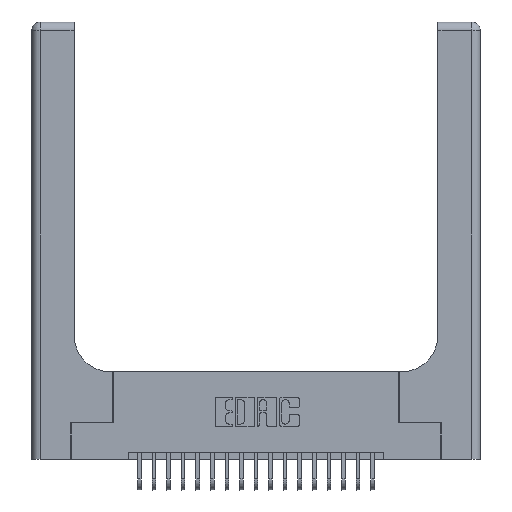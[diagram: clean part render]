
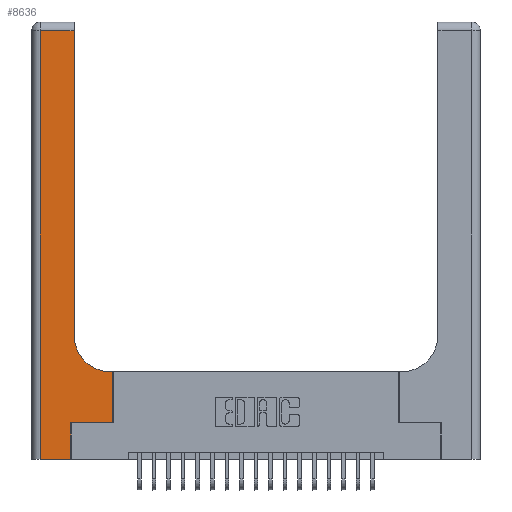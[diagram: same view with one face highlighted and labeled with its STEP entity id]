
A CAD part, top view. The second image highlights one B-rep face of the part: STEP entity #8636.
In plain terms, the highlighted planar face has unit normal (0, 0, 1).
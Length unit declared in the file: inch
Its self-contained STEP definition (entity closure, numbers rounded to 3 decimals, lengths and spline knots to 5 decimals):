
#656 = EDGE_CURVE ( 'NONE', #9086, #6946, #1847, .T. ) ;
#853 = VERTEX_POINT ( 'NONE', #21375 ) ;
#895 = CARTESIAN_POINT ( 'NONE',  ( 0.269, 0., 0.37 ) ) ;
#916 = LINE ( 'NONE', #15153, #19738 ) ;
#1081 = LINE ( 'NONE', #7070, #23276 ) ;
#1116 = VERTEX_POINT ( 'NONE', #2215 ) ;
#1467 = VECTOR ( 'NONE', #8003, 39.37008 ) ;
#1506 = VECTOR ( 'NONE', #14031, 39.37008 ) ;
#1847 = LINE ( 'NONE', #6470, #15522 ) ;
#2215 = CARTESIAN_POINT ( 'NONE',  ( 0.2915, 2.94, 0.37 ) ) ;
#2321 = DIRECTION ( 'NONE',  ( 0., 0., -1. ) ) ;
#2391 = DIRECTION ( 'NONE',  ( 0., 0., -1. ) ) ;
#2505 = EDGE_CURVE ( 'NONE', #12553, #1116, #916, .T. ) ;
#2933 = LINE ( 'NONE', #3428, #1506 ) ;
#3012 = ORIENTED_EDGE ( 'NONE', *, *, #11984, .T. ) ;
#3163 = EDGE_CURVE ( 'NONE', #1116, #22739, #12796, .T. ) ;
#3407 = CARTESIAN_POINT ( 'NONE',  ( 0.2915, 0.85, 0.37 ) ) ;
#3428 = CARTESIAN_POINT ( 'NONE',  ( 0., 0., 0.37 ) ) ;
#4200 = CARTESIAN_POINT ( 'NONE',  ( 0.5585, 0.25, 0.37 ) ) ;
#4352 = EDGE_CURVE ( 'NONE', #22739, #20454, #1081, .T. ) ;
#4397 = LINE ( 'NONE', #4946, #15492 ) ;
#4946 = CARTESIAN_POINT ( 'NONE',  ( 0.2915, 0.6, 0.37 ) ) ;
#6448 = ORIENTED_EDGE ( 'NONE', *, *, #22665, .T. ) ;
#6470 = CARTESIAN_POINT ( 'NONE',  ( 0.269, 0.25, 0.37 ) ) ;
#6734 = CARTESIAN_POINT ( 'NONE',  ( 0., 2.94, 0.37 ) ) ;
#6946 = VERTEX_POINT ( 'NONE', #21817 ) ;
#7070 = CARTESIAN_POINT ( 'NONE',  ( 0.06, 3., 0.37 ) ) ;
#7709 = LINE ( 'NONE', #4200, #1467 ) ;
#7844 = CARTESIAN_POINT ( 'NONE',  ( 0.269, 0., 0.37 ) ) ;
#7920 = EDGE_CURVE ( 'NONE', #6946, #853, #7709, .T. ) ;
#8003 = DIRECTION ( 'NONE',  ( 0., 1., 0. ) ) ;
#8152 = AXIS2_PLACEMENT_3D ( 'NONE', #13316, #2391, #16904 ) ;
#8636 = ADVANCED_FACE ( 'NONE', ( #13153 ), #13398, .F. ) ;
#8819 = DIRECTION ( 'NONE',  ( 0., -1., 0. ) ) ;
#9086 = VERTEX_POINT ( 'NONE', #16178 ) ;
#9945 = VERTEX_POINT ( 'NONE', #16929 ) ;
#10092 = CIRCLE ( 'NONE', #14457, 0.25 ) ;
#10537 = ORIENTED_EDGE ( 'NONE', *, *, #7920, .T. ) ;
#10909 = CARTESIAN_POINT ( 'NONE',  ( 0.06, 2.94, 0.37 ) ) ;
#11194 = DIRECTION ( 'NONE',  ( 1., 0., 0. ) ) ;
#11984 = EDGE_CURVE ( 'NONE', #20454, #20222, #2933, .T. ) ;
#12553 = VERTEX_POINT ( 'NONE', #3407 ) ;
#12619 = ORIENTED_EDGE ( 'NONE', *, *, #4352, .T. ) ;
#12796 = LINE ( 'NONE', #6734, #16226 ) ;
#13107 = EDGE_LOOP ( 'NONE', ( #14057, #20870, #12619, #3012, #14576, #21578, #10537, #6448, #15050 ) ) ;
#13153 = FACE_OUTER_BOUND ( 'NONE', #13107, .T. ) ;
#13316 = CARTESIAN_POINT ( 'NONE',  ( 0., 3., 0.37 ) ) ;
#13398 = PLANE ( 'NONE',  #8152 ) ;
#14031 = DIRECTION ( 'NONE',  ( 1., 0., 0. ) ) ;
#14057 = ORIENTED_EDGE ( 'NONE', *, *, #2505, .T. ) ;
#14151 = EDGE_CURVE ( 'NONE', #20222, #9086, #19675, .T. ) ;
#14457 = AXIS2_PLACEMENT_3D ( 'NONE', #18667, #2321, #11194 ) ;
#14576 = ORIENTED_EDGE ( 'NONE', *, *, #14151, .T. ) ;
#15050 = ORIENTED_EDGE ( 'NONE', *, *, #22252, .T. ) ;
#15153 = CARTESIAN_POINT ( 'NONE',  ( 0.2915, 3., 0.37 ) ) ;
#15492 = VECTOR ( 'NONE', #17702, 39.37008 ) ;
#15522 = VECTOR ( 'NONE', #22876, 39.37008 ) ;
#16178 = CARTESIAN_POINT ( 'NONE',  ( 0.269, 0.25, 0.37 ) ) ;
#16226 = VECTOR ( 'NONE', #17577, 39.37008 ) ;
#16904 = DIRECTION ( 'NONE',  ( -1., 0., 0. ) ) ;
#16929 = CARTESIAN_POINT ( 'NONE',  ( 0.5415, 0.6, 0.37 ) ) ;
#17378 = VECTOR ( 'NONE', #19132, 39.37008 ) ;
#17577 = DIRECTION ( 'NONE',  ( -1., 0., 0. ) ) ;
#17702 = DIRECTION ( 'NONE',  ( -1., 0., 0. ) ) ;
#18111 = CARTESIAN_POINT ( 'NONE',  ( 0.06, 0., 0.37 ) ) ;
#18667 = CARTESIAN_POINT ( 'NONE',  ( 0.5415, 0.85, 0.37 ) ) ;
#18822 = DIRECTION ( 'NONE',  ( 0., 1., 0. ) ) ;
#19132 = DIRECTION ( 'NONE',  ( 0., 1., 0. ) ) ;
#19675 = LINE ( 'NONE', #895, #17378 ) ;
#19738 = VECTOR ( 'NONE', #18822, 39.37008 ) ;
#20222 = VERTEX_POINT ( 'NONE', #7844 ) ;
#20454 = VERTEX_POINT ( 'NONE', #18111 ) ;
#20870 = ORIENTED_EDGE ( 'NONE', *, *, #3163, .T. ) ;
#21375 = CARTESIAN_POINT ( 'NONE',  ( 0.5585, 0.6, 0.37 ) ) ;
#21578 = ORIENTED_EDGE ( 'NONE', *, *, #656, .T. ) ;
#21817 = CARTESIAN_POINT ( 'NONE',  ( 0.5585, 0.25, 0.37 ) ) ;
#22252 = EDGE_CURVE ( 'NONE', #9945, #12553, #10092, .T. ) ;
#22665 = EDGE_CURVE ( 'NONE', #853, #9945, #4397, .T. ) ;
#22739 = VERTEX_POINT ( 'NONE', #10909 ) ;
#22876 = DIRECTION ( 'NONE',  ( 1., 0., 0. ) ) ;
#23276 = VECTOR ( 'NONE', #8819, 39.37008 ) ;
